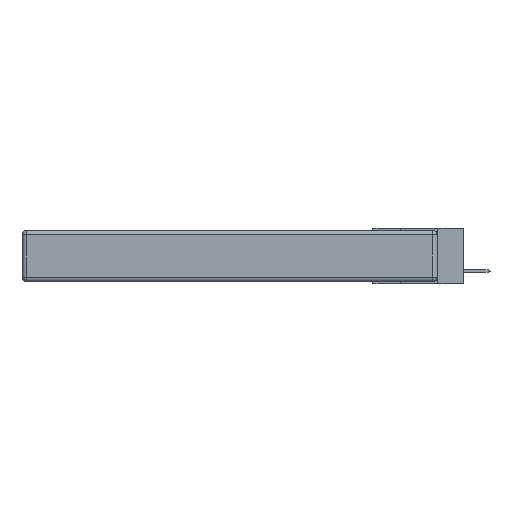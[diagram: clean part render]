
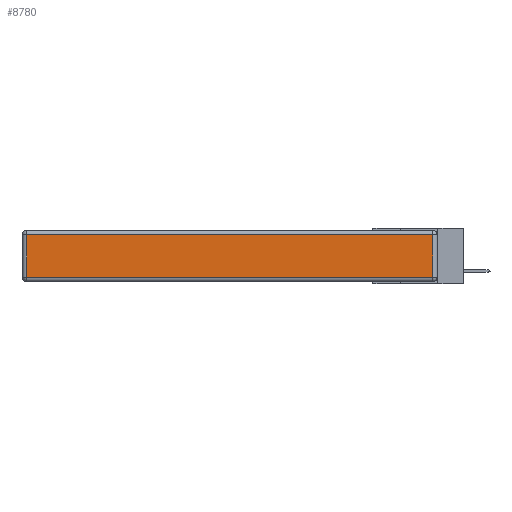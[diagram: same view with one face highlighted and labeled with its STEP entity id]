
A CAD part, left-side view. The second image highlights one B-rep face of the part: STEP entity #8780.
In plain terms, the highlighted planar face has unit normal (-1, 0, 0).
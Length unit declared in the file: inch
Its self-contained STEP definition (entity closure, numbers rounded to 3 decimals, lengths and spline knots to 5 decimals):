
#145 = ORIENTED_EDGE ( 'NONE', *, *, #7007, .T. ) ;
#904 = LINE ( 'NONE', #6573, #20782 ) ;
#1082 = FACE_OUTER_BOUND ( 'NONE', #21900, .T. ) ;
#3116 = LINE ( 'NONE', #8713, #14025 ) ;
#3224 = ORIENTED_EDGE ( 'NONE', *, *, #16584, .T. ) ;
#3910 = CARTESIAN_POINT ( 'NONE',  ( 0., 0., -0.343 ) ) ;
#4964 = ORIENTED_EDGE ( 'NONE', *, *, #20213, .T. ) ;
#6238 = CARTESIAN_POINT ( 'NONE',  ( 0., 2.72, -0.03 ) ) ;
#6573 = CARTESIAN_POINT ( 'NONE',  ( 0., 2.75, -0.03 ) ) ;
#7007 = EDGE_CURVE ( 'NONE', #16984, #11890, #13951, .T. ) ;
#7223 = VERTEX_POINT ( 'NONE', #10124 ) ;
#7383 = DIRECTION ( 'NONE',  ( -1., 0., 0. ) ) ;
#8063 = DIRECTION ( 'NONE',  ( 0., 0., -1. ) ) ;
#8484 = VERTEX_POINT ( 'NONE', #6238 ) ;
#8713 = CARTESIAN_POINT ( 'NONE',  ( 0., 0.03, -0.343 ) ) ;
#8780 = ADVANCED_FACE ( 'NONE', ( #1082 ), #8881, .T. ) ;
#8881 = PLANE ( 'NONE',  #19098 ) ;
#10124 = CARTESIAN_POINT ( 'NONE',  ( 0., 0.03, -0.03 ) ) ;
#10357 = DIRECTION ( 'NONE',  ( 0., 0., 1. ) ) ;
#10528 = DIRECTION ( 'NONE',  ( 0., 0., 1. ) ) ;
#11186 = CARTESIAN_POINT ( 'NONE',  ( 0., 0., -0.313 ) ) ;
#11200 = VECTOR ( 'NONE', #8063, 39.37008 ) ;
#11890 = VERTEX_POINT ( 'NONE', #12584 ) ;
#12584 = CARTESIAN_POINT ( 'NONE',  ( 0., 0.03, -0.313 ) ) ;
#13107 = VECTOR ( 'NONE', #21439, 39.37008 ) ;
#13951 = LINE ( 'NONE', #11186, #13107 ) ;
#14025 = VECTOR ( 'NONE', #10357, 39.37008 ) ;
#14447 = EDGE_CURVE ( 'NONE', #7223, #8484, #904, .T. ) ;
#16584 = EDGE_CURVE ( 'NONE', #11890, #7223, #3116, .T. ) ;
#16721 = ORIENTED_EDGE ( 'NONE', *, *, #14447, .T. ) ;
#16984 = VERTEX_POINT ( 'NONE', #19950 ) ;
#19098 = AXIS2_PLACEMENT_3D ( 'NONE', #3910, #7383, #10528 ) ;
#19950 = CARTESIAN_POINT ( 'NONE',  ( 0., 2.72, -0.313 ) ) ;
#20137 = DIRECTION ( 'NONE',  ( 0., 1., 0. ) ) ;
#20203 = LINE ( 'NONE', #21435, #11200 ) ;
#20213 = EDGE_CURVE ( 'NONE', #8484, #16984, #20203, .T. ) ;
#20782 = VECTOR ( 'NONE', #20137, 39.37008 ) ;
#21435 = CARTESIAN_POINT ( 'NONE',  ( 0., 2.72, -0.343 ) ) ;
#21439 = DIRECTION ( 'NONE',  ( 0., -1., 0. ) ) ;
#21900 = EDGE_LOOP ( 'NONE', ( #145, #3224, #16721, #4964 ) ) ;
